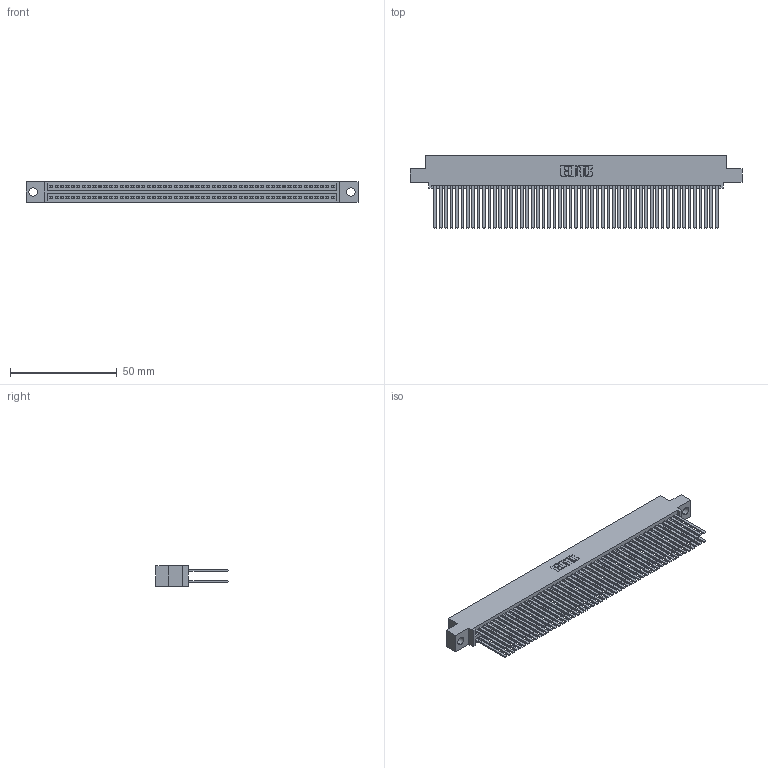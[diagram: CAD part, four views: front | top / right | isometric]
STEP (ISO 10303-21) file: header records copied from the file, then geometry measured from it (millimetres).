
FILE_DESCRIPTION (( 'STEP AP203' ), '1' );
FILE_NAME ('345-106-544-504.STEP', '2021-05-21T14:08:42', ( '' ), ( '' ), 'SwSTEP 2.0', 'SolidWorks 2020', '' );
FILE_SCHEMA (( 'CONFIG_CONTROL_DESIGN' ));
Length unit declared in the file: inch
Products named in the file (3): 345-106-544-504; 345 Part_0.110 Offset - 0.156 Dia-TI; 345-292-001_345-293-144
Assembly tree (107 placements, depth 2):
  345-106-544-504
    345 Part_0.110 Offset - 0.156 Dia-TI
    345-292-001_345-293-144  x106
Bounding box: 155.83 x 33.96 x 9.4 mm (x, y, z)
Volume: 16546.1 mm3; surface area: 28970.5 mm2
Topology: 107 solids, 107 shells, 4808 faces, 14275 edges, 9374 vertices
Faces by surface type: plane 3172, cylinder 1636
Entity records: 40471 total; most frequent: CARTESIAN_POINT 6778, ORIENTED_EDGE 6710, DIRECTION 5959, EDGE_CURVE 3355, VECTOR 3015, LINE 3015, VERTEX_POINT 2234, AXIS2_PLACEMENT_3D 1472
